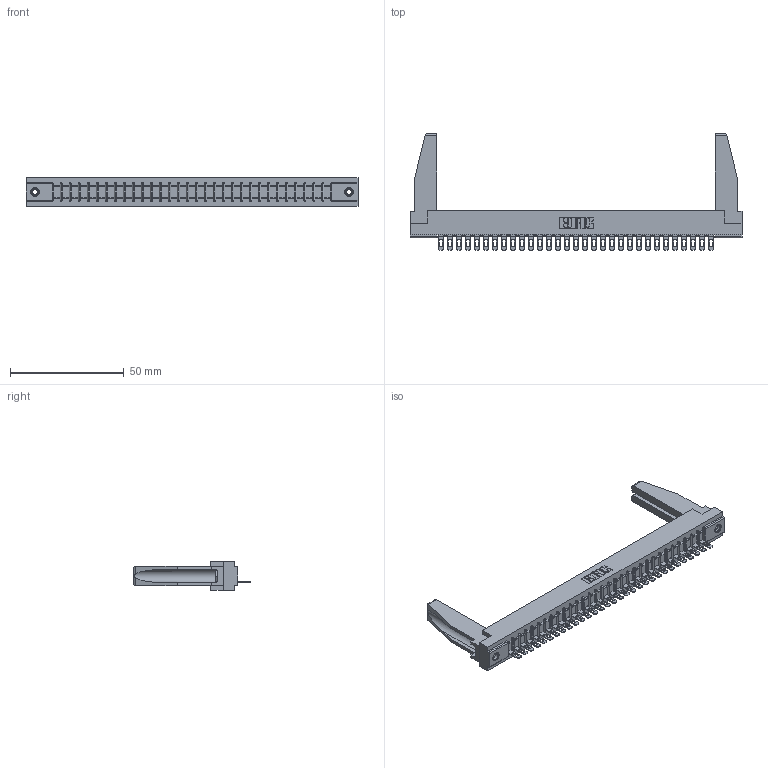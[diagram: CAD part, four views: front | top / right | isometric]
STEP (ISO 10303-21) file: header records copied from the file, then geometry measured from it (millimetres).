
FILE_DESCRIPTION (( 'STEP AP203' ), '1' );
FILE_NAME ('357-031-501-178.STEP', '2019-09-17T03:35:30', ( '' ), ( '' ), 'SwSTEP 2.0', 'SolidWorks 2016', '' );
FILE_SCHEMA (( 'CONFIG_CONTROL_DESIGN' ));
Length unit declared in the file: inch
Products named in the file (5): 307 Part_.156 Dia Mounting Holes; 307-290-002_501; 345-250-001_345-250-001-102; 307-220-078; 357-031-501-178
Assembly tree (36 placements, depth 2):
  357-031-501-178
    307 Part_.156 Dia Mounting Holes
    307-290-002_501  x31
    307-220-078  x2
    345-250-001_345-250-001-102  x2
Bounding box: 145.85 x 51.13 x 12.7 mm (x, y, z)
Volume: 19545.8 mm3; surface area: 23348.9 mm2
Topology: 36 solids, 36 shells, 2636 faces, 8031 edges, 5258 vertices
Faces by surface type: plane 1518, cylinder 1038, sphere 64, cone 12, torus 4
Entity records: 31165 total; most frequent: CARTESIAN_POINT 5254, ORIENTED_EDGE 5200, DIRECTION 5070, EDGE_CURVE 2600, LINE 1986, VECTOR 1986, VERTEX_POINT 1684, AXIS2_PLACEMENT_3D 1542
